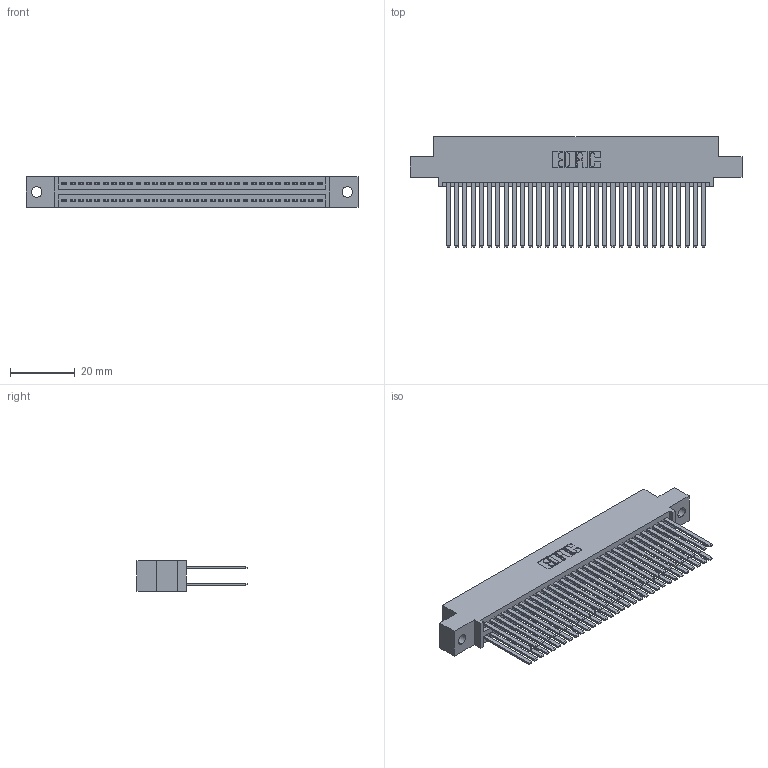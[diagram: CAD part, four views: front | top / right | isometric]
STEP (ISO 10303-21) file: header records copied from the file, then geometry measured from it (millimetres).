
FILE_DESCRIPTION (( 'STEP AP203' ), '1' );
FILE_NAME ('345-064-544-502.STEP', '2019-10-30T14:34:56', ( '' ), ( '' ), 'SwSTEP 2.0', 'SolidWorks 2016', '' );
FILE_SCHEMA (( 'CONFIG_CONTROL_DESIGN' ));
Length unit declared in the file: inch
Products named in the file (3): 345-292-001_345-293-144; 345 Part_0.110 Offset - 0.128 Dia; 345-064-544-502
Assembly tree (65 placements, depth 2):
  345-064-544-502
    345 Part_0.110 Offset - 0.128 Dia
    345-292-001_345-293-144  x64
Bounding box: 102.49 x 33.96 x 9.4 mm (x, y, z)
Volume: 10650.2 mm3; surface area: 17998.7 mm2
Topology: 65 solids, 65 shells, 2946 faces, 8737 edges, 5738 vertices
Faces by surface type: plane 1940, cylinder 1006
Entity records: 26405 total; most frequent: CARTESIAN_POINT 4436, ORIENTED_EDGE 4370, DIRECTION 3921, EDGE_CURVE 2185, VECTOR 1929, LINE 1929, VERTEX_POINT 1454, AXIS2_PLACEMENT_3D 996
